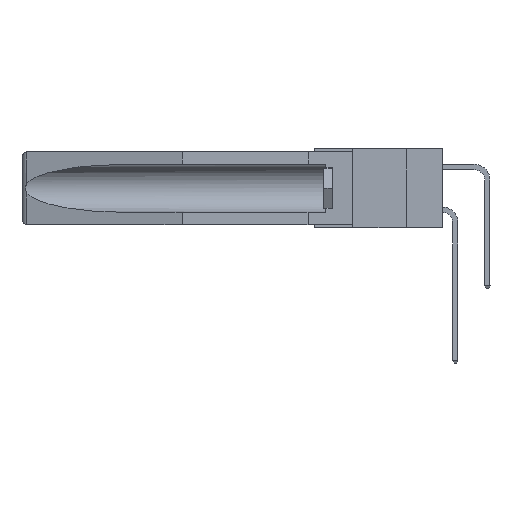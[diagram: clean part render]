
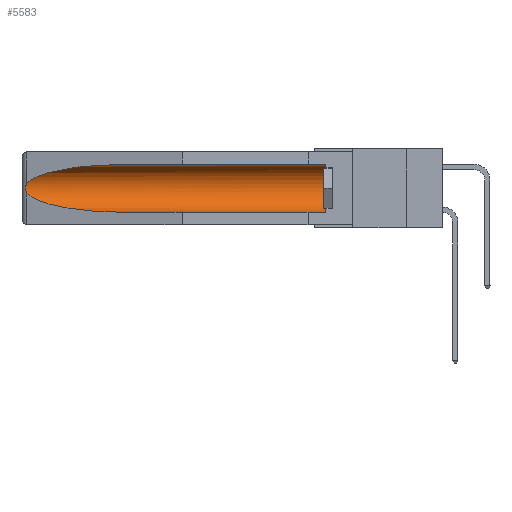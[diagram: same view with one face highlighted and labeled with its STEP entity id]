
A CAD part, left-side view. The second image highlights one B-rep face of the part: STEP entity #5583.
In plain terms, the highlighted cylindrical face has radius 2.857 mm (diameter 5.715 mm), a partial arc.
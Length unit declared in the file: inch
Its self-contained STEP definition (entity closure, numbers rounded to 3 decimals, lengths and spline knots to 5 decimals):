
#1014 = VERTEX_POINT ( 'NONE', #15767 ) ;
#1132 = ORIENTED_EDGE ( 'NONE', *, *, #5273, .T. ) ;
#1534 = CARTESIAN_POINT ( 'NONE',  ( 0.21114, 1.30732, -0.284 ) ) ;
#2059 = LINE ( 'NONE', #20166, #4867 ) ;
#2363 = ORIENTED_EDGE ( 'NONE', *, *, #12325, .T. ) ;
#2653 = CARTESIAN_POINT ( 'NONE',  ( 0.26597, 1.5296, -0.19026 ) ) ;
#3041 = CARTESIAN_POINT ( 'NONE',  ( 0.155, 1.07973, -0.284 ) ) ;
#3289 = ORIENTED_EDGE ( 'NONE', *, *, #8652, .T. ) ;
#4034 = EDGE_LOOP ( 'NONE', ( #3289, #1132, #14551, #20146, #11081, #2363 ) ) ;
#4557 = VERTEX_POINT ( 'NONE', #14175 ) ;
#4816 = CARTESIAN_POINT ( 'NONE',  ( 0.155, -0.30754, -0.1715 ) ) ;
#4867 = VECTOR ( 'NONE', #5496, 39.37008 ) ;
#4883 = DIRECTION ( 'NONE',  ( 0., 1., 0. ) ) ;
#5273 = EDGE_CURVE ( 'NONE', #12949, #13570, #12422, .T. ) ;
#5496 = DIRECTION ( 'NONE',  ( 0., 1., 0. ) ) ;
#5583 = ADVANCED_FACE ( 'NONE', ( #12420 ), #7784, .F. ) ;
#5614 = CARTESIAN_POINT ( 'NONE',  ( 0.155, 1.07973, -0.059 ) ) ;
#5640 = DIRECTION ( 'NONE',  ( 0., 1., 0. ) ) ;
#5924 = CARTESIAN_POINT ( 'NONE',  ( 0.26537, 1.52718, -0.14972 ) ) ;
#6106 = EDGE_CURVE ( 'NONE', #4557, #19144, #2059, .T. ) ;
#6842 = AXIS2_PLACEMENT_3D ( 'NONE', #4816, #4883, #13021 ) ;
#7069 = LINE ( 'NONE', #10594, #9642 ) ;
#7103 = CARTESIAN_POINT ( 'NONE',  ( 0.2675, 1.53308, -0.17534 ) ) ;
#7547 = CARTESIAN_POINT ( 'NONE',  ( 0.25451, 1.48313, -0.09465 ) ) ;
#7621 = CARTESIAN_POINT ( 'NONE',  ( 0.2673, 1.53269, -0.17917 ) ) ;
#7707 = CARTESIAN_POINT ( 'NONE',  ( 0.25451, 1.48313, -0.24835 ) ) ;
#7784 = CYLINDRICAL_SURFACE ( 'NONE', #6842, 0.1125 ) ;
#8652 = EDGE_CURVE ( 'NONE', #16072, #12949, #13084, .T. ) ;
#9642 = VECTOR ( 'NONE', #5640, 39.37008 ) ;
#10409 = DIRECTION ( 'NONE',  ( 0., 0., 1. ) ) ;
#10485 = CARTESIAN_POINT ( 'NONE',  ( 0.26597, 1.52961, -0.15275 ) ) ;
#10594 = CARTESIAN_POINT ( 'NONE',  ( 0.155, -0.30754, -0.059 ) ) ;
#11081 = ORIENTED_EDGE ( 'NONE', *, *, #14264, .T. ) ;
#11227 = AXIS2_PLACEMENT_3D ( 'NONE', #18510, #13809, #10409 ) ;
#11620 = CIRCLE ( 'NONE', #11227, 0.1125 ) ;
#12268 = CARTESIAN_POINT ( 'NONE',  ( 0.155, 1.07973, -0.059 ) ) ;
#12325 = EDGE_CURVE ( 'NONE', #1014, #16072, #7069, .T. ) ;
#12420 = FACE_OUTER_BOUND ( 'NONE', #4034, .T. ) ;
#12422 = B_SPLINE_CURVE_WITH_KNOTS ( 'NONE', 3,
 ( #5924, #10485, #17001, #15313, #12590, #7103, #7621, #17610, #2653, #17152 ),
 .UNSPECIFIED., .F., .F.,
 ( 4, 2, 2, 2, 4 ),
 ( 0., 0.00029, 0.00058, 0.00087, 0.00117 ),
 .UNSPECIFIED. ) ;
#12590 = CARTESIAN_POINT ( 'NONE',  ( 0.2675, 1.53308, -0.16763 ) ) ;
#12949 = VERTEX_POINT ( 'NONE', #19813 ) ;
#13021 = DIRECTION ( 'NONE',  ( 0., 0., 1. ) ) ;
#13084 =( BOUNDED_CURVE ( )  B_SPLINE_CURVE ( 3, ( #5614, #17384, #7547, #17226 ),
 .UNSPECIFIED., .F., .F. ) 
 B_SPLINE_CURVE_WITH_KNOTS ( ( 4, 4 ),
 ( 4.71239, 6.08839 ),
 .UNSPECIFIED. ) 
 CURVE ( )  GEOMETRIC_REPRESENTATION_ITEM ( )  RATIONAL_B_SPLINE_CURVE ( ( 1., 0.848, 0.848, 1. ) ) 
 REPRESENTATION_ITEM ( '' )  );
#13556 = EDGE_CURVE ( 'NONE', #13570, #19144, #21177, .T. ) ;
#13570 = VERTEX_POINT ( 'NONE', #19278 ) ;
#13809 = DIRECTION ( 'NONE',  ( 0., -1., 0. ) ) ;
#14175 = CARTESIAN_POINT ( 'NONE',  ( 0.155, 0.126, -0.284 ) ) ;
#14264 = EDGE_CURVE ( 'NONE', #4557, #1014, #11620, .T. ) ;
#14551 = ORIENTED_EDGE ( 'NONE', *, *, #13556, .T. ) ;
#15313 = CARTESIAN_POINT ( 'NONE',  ( 0.2673, 1.5327, -0.16383 ) ) ;
#15767 = CARTESIAN_POINT ( 'NONE',  ( 0.155, 0.126, -0.059 ) ) ;
#16072 = VERTEX_POINT ( 'NONE', #12268 ) ;
#17001 = CARTESIAN_POINT ( 'NONE',  ( 0.26654, 1.53092, -0.15636 ) ) ;
#17152 = CARTESIAN_POINT ( 'NONE',  ( 0.26537, 1.52718, -0.19328 ) ) ;
#17226 = CARTESIAN_POINT ( 'NONE',  ( 0.26537, 1.52718, -0.14972 ) ) ;
#17384 = CARTESIAN_POINT ( 'NONE',  ( 0.21114, 1.30732, -0.059 ) ) ;
#17610 = CARTESIAN_POINT ( 'NONE',  ( 0.26655, 1.53094, -0.18657 ) ) ;
#18510 = CARTESIAN_POINT ( 'NONE',  ( 0.155, 0.126, -0.1715 ) ) ;
#19144 = VERTEX_POINT ( 'NONE', #19971 ) ;
#19278 = CARTESIAN_POINT ( 'NONE',  ( 0.26537, 1.52718, -0.19328 ) ) ;
#19813 = CARTESIAN_POINT ( 'NONE',  ( 0.26537, 1.52718, -0.14972 ) ) ;
#19971 = CARTESIAN_POINT ( 'NONE',  ( 0.155, 1.07973, -0.284 ) ) ;
#20146 = ORIENTED_EDGE ( 'NONE', *, *, #6106, .F. ) ;
#20166 = CARTESIAN_POINT ( 'NONE',  ( 0.155, -0.30754, -0.284 ) ) ;
#20894 = CARTESIAN_POINT ( 'NONE',  ( 0.26537, 1.52718, -0.19328 ) ) ;
#21177 =( BOUNDED_CURVE ( )  B_SPLINE_CURVE ( 3, ( #20894, #7707, #1534, #3041 ),
 .UNSPECIFIED., .F., .T. ) 
 B_SPLINE_CURVE_WITH_KNOTS ( ( 4, 4 ),
 ( 0.1948, 1.5708 ),
 .UNSPECIFIED. ) 
 CURVE ( )  GEOMETRIC_REPRESENTATION_ITEM ( )  RATIONAL_B_SPLINE_CURVE ( ( 1., 0.848, 0.848, 1. ) ) 
 REPRESENTATION_ITEM ( '' )  );
